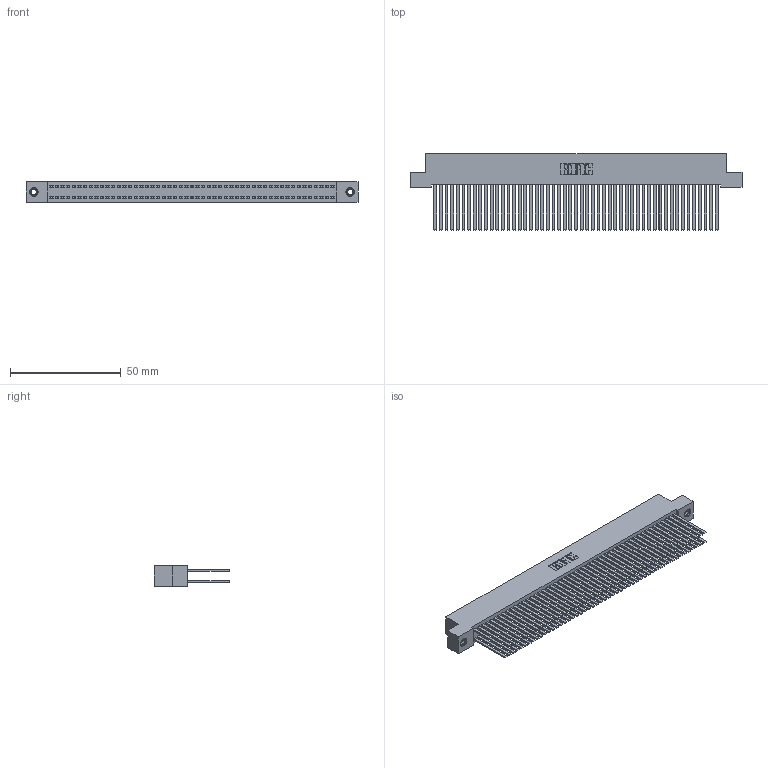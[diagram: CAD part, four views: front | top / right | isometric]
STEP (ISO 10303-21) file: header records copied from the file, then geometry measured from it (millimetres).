
FILE_DESCRIPTION (( 'STEP AP203' ), '1' );
FILE_NAME ('342-102-544-207.STEP', '2019-10-04T18:16:02', ( '' ), ( '' ), 'SwSTEP 2.0', 'SolidWorks 2016', '' );
FILE_SCHEMA (( 'CONFIG_CONTROL_DESIGN' ));
Length unit declared in the file: inch
Products named in the file (4): 342 Part_TI; 345-292-001_345-293-144; 345-250-001_345-250-005-103; 342-102-544-207
Assembly tree (105 placements, depth 2):
  342-102-544-207
    342 Part_TI
    345-292-001_345-293-144  x102
    345-250-001_345-250-005-103  x2
Bounding box: 149.86 x 34.3 x 9.4 mm (x, y, z)
Volume: 14924.7 mm3; surface area: 28500.9 mm2
Topology: 105 solids, 105 shells, 4862 faces, 14409 edges, 9462 vertices
Faces by surface type: plane 3362, cylinder 1484, cone 12, torus 4
Entity records: 32516 total; most frequent: CARTESIAN_POINT 5357, ORIENTED_EDGE 5286, DIRECTION 4589, EDGE_CURVE 2643, LINE 2499, VECTOR 2499, VERTEX_POINT 1756, AXIS2_PLACEMENT_3D 1045
